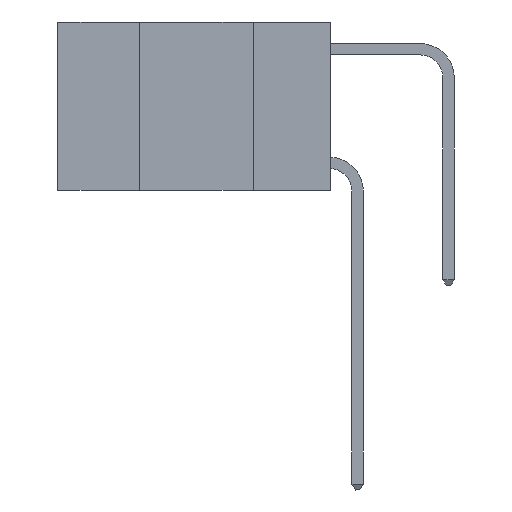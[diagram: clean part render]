
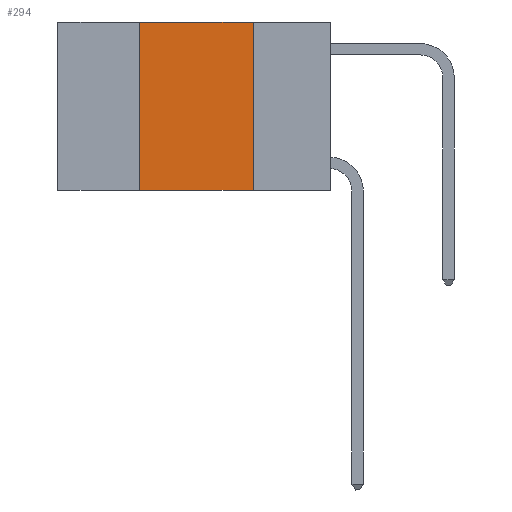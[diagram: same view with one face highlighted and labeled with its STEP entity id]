
A CAD part, left-side view. The second image highlights one B-rep face of the part: STEP entity #294.
In plain terms, the highlighted planar face has unit normal (-1, 0, 0).
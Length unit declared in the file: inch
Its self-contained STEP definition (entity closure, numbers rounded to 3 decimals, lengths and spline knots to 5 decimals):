
#201 = CARTESIAN_POINT ( 'NONE',  ( 0., 0.42, 0. ) ) ;
#294 = ADVANCED_FACE ( 'NONE', ( #8871 ), #6240, .F. ) ;
#999 = DIRECTION ( 'NONE',  ( 0., 0., 1. ) ) ;
#1275 = VECTOR ( 'NONE', #999, 39.37008 ) ;
#2115 = CARTESIAN_POINT ( 'NONE',  ( 0., 0.17, 0. ) ) ;
#2463 = VERTEX_POINT ( 'NONE', #201 ) ;
#2788 = VECTOR ( 'NONE', #15009, 39.37008 ) ;
#4254 = LINE ( 'NONE', #15140, #1275 ) ;
#4375 = ORIENTED_EDGE ( 'NONE', *, *, #10263, .F. ) ;
#4383 = VECTOR ( 'NONE', #11305, 39.37008 ) ;
#4438 = ORIENTED_EDGE ( 'NONE', *, *, #8522, .T. ) ;
#4586 = VERTEX_POINT ( 'NONE', #9280 ) ;
#4710 = EDGE_CURVE ( 'NONE', #2463, #5897, #10084, .T. ) ;
#5639 = DIRECTION ( 'NONE',  ( 1., 0., 0. ) ) ;
#5897 = VERTEX_POINT ( 'NONE', #8794 ) ;
#6008 = LINE ( 'NONE', #2115, #2788 ) ;
#6033 = DIRECTION ( 'NONE',  ( 0., -1., 0. ) ) ;
#6240 = PLANE ( 'NONE',  #10151 ) ;
#7022 = VECTOR ( 'NONE', #6033, 39.37008 ) ;
#7804 = CARTESIAN_POINT ( 'NONE',  ( 0., 0.6, -0.37 ) ) ;
#8522 = EDGE_CURVE ( 'NONE', #4586, #8619, #11824, .T. ) ;
#8619 = VERTEX_POINT ( 'NONE', #13755 ) ;
#8794 = CARTESIAN_POINT ( 'NONE',  ( 0., 0.17, 0. ) ) ;
#8871 = FACE_OUTER_BOUND ( 'NONE', #10216, .T. ) ;
#9280 = CARTESIAN_POINT ( 'NONE',  ( 0., 0.42, -0.37 ) ) ;
#10084 = LINE ( 'NONE', #11800, #7022 ) ;
#10151 = AXIS2_PLACEMENT_3D ( 'NONE', #10726, #5639, #15273 ) ;
#10216 = EDGE_LOOP ( 'NONE', ( #4375, #11723, #13290, #4438 ) ) ;
#10263 = EDGE_CURVE ( 'NONE', #5897, #8619, #6008, .T. ) ;
#10726 = CARTESIAN_POINT ( 'NONE',  ( 0., 0.6, 0. ) ) ;
#11305 = DIRECTION ( 'NONE',  ( 0., -1., 0. ) ) ;
#11723 = ORIENTED_EDGE ( 'NONE', *, *, #4710, .F. ) ;
#11800 = CARTESIAN_POINT ( 'NONE',  ( 0., 0.6, 0. ) ) ;
#11824 = LINE ( 'NONE', #7804, #4383 ) ;
#13290 = ORIENTED_EDGE ( 'NONE', *, *, #15202, .F. ) ;
#13755 = CARTESIAN_POINT ( 'NONE',  ( 0., 0.17, -0.37 ) ) ;
#15009 = DIRECTION ( 'NONE',  ( 0., 0., -1. ) ) ;
#15140 = CARTESIAN_POINT ( 'NONE',  ( 0., 0.42, 0. ) ) ;
#15202 = EDGE_CURVE ( 'NONE', #4586, #2463, #4254, .T. ) ;
#15273 = DIRECTION ( 'NONE',  ( 0., 0., -1. ) ) ;
